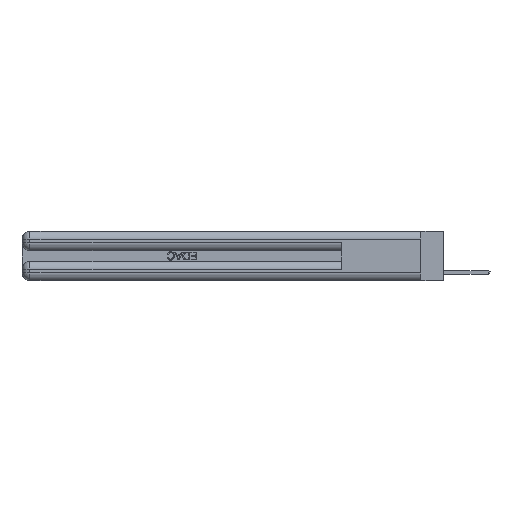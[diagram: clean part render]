
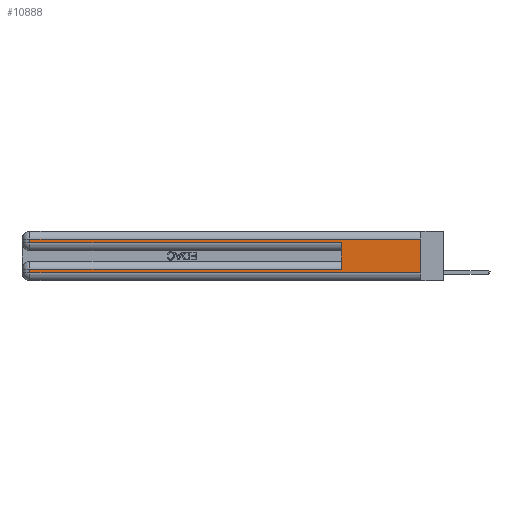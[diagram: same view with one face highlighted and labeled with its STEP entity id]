
A CAD part, left-side view. The second image highlights one B-rep face of the part: STEP entity #10888.
In plain terms, the highlighted planar face has unit normal (-1, 0, 0).
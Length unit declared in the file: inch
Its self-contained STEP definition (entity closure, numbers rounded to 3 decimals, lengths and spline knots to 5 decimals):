
#2613 = ORIENTED_EDGE ( 'NONE', *, *, #18025, .T. ) ;
#2852 = CARTESIAN_POINT ( 'NONE',  ( 0., 0., 0.31 ) ) ;
#3670 = VERTEX_POINT ( 'NONE', #18301 ) ;
#3896 = CARTESIAN_POINT ( 'NONE',  ( 0., 0., 0.31 ) ) ;
#4513 = VECTOR ( 'NONE', #7351, 39.37008 ) ;
#4706 = FACE_OUTER_BOUND ( 'NONE', #17770, .T. ) ;
#5060 = CARTESIAN_POINT ( 'NONE',  ( 0., 0., 0.06 ) ) ;
#5392 = VERTEX_POINT ( 'NONE', #24431 ) ;
#6036 = VERTEX_POINT ( 'NONE', #26670 ) ;
#6411 = VERTEX_POINT ( 'NONE', #17900 ) ;
#6585 = CARTESIAN_POINT ( 'NONE',  ( 0., 0.6, 0.145 ) ) ;
#7351 = DIRECTION ( 'NONE',  ( 0., 0., -1. ) ) ;
#8459 = ORIENTED_EDGE ( 'NONE', *, *, #19089, .F. ) ;
#9196 = CARTESIAN_POINT ( 'NONE',  ( 0., 2.94, 0.085 ) ) ;
#10409 = DIRECTION ( 'NONE',  ( 0., 0., -1. ) ) ;
#10888 = ADVANCED_FACE ( 'NONE', ( #4706 ), #28936, .F. ) ;
#11468 = LINE ( 'NONE', #24346, #15076 ) ;
#11641 = DIRECTION ( 'NONE',  ( 0., -1., 0. ) ) ;
#11664 = EDGE_CURVE ( 'NONE', #6036, #26321, #22781, .T. ) ;
#12719 = VECTOR ( 'NONE', #18412, 39.37008 ) ;
#12930 = AXIS2_PLACEMENT_3D ( 'NONE', #17238, #15119, #26695 ) ;
#13207 = ORIENTED_EDGE ( 'NONE', *, *, #11664, .T. ) ;
#13581 = LINE ( 'NONE', #27508, #18640 ) ;
#13871 = VECTOR ( 'NONE', #19213, 39.37008 ) ;
#14738 = CARTESIAN_POINT ( 'NONE',  ( 0., 2.94, 0.37 ) ) ;
#15076 = VECTOR ( 'NONE', #10409, 39.37008 ) ;
#15119 = DIRECTION ( 'NONE',  ( 1., 0., 0. ) ) ;
#16071 = ORIENTED_EDGE ( 'NONE', *, *, #19664, .T. ) ;
#16158 = EDGE_CURVE ( 'NONE', #26321, #28651, #26924, .T. ) ;
#16283 = VERTEX_POINT ( 'NONE', #20315 ) ;
#16354 = ORIENTED_EDGE ( 'NONE', *, *, #24091, .T. ) ;
#16375 = ORIENTED_EDGE ( 'NONE', *, *, #16158, .T. ) ;
#17210 = DIRECTION ( 'NONE',  ( 0., 1., 0. ) ) ;
#17238 = CARTESIAN_POINT ( 'NONE',  ( 0., 0., 0.37 ) ) ;
#17770 = EDGE_LOOP ( 'NONE', ( #19878, #16071, #16354, #28757, #8459, #13207, #16375, #2613 ) ) ;
#17900 = CARTESIAN_POINT ( 'NONE',  ( 0., 2.94, 0.285 ) ) ;
#18025 = EDGE_CURVE ( 'NONE', #28651, #16283, #19269, .T. ) ;
#18301 = CARTESIAN_POINT ( 'NONE',  ( 0., 0.6, 0.285 ) ) ;
#18412 = DIRECTION ( 'NONE',  ( 0., 0., 1. ) ) ;
#18640 = VECTOR ( 'NONE', #23364, 39.37008 ) ;
#19089 = EDGE_CURVE ( 'NONE', #6036, #3670, #21743, .T. ) ;
#19213 = DIRECTION ( 'NONE',  ( 0., 1., 0. ) ) ;
#19269 = LINE ( 'NONE', #5060, #20688 ) ;
#19350 = DIRECTION ( 'NONE',  ( 0., -1., 0. ) ) ;
#19601 = VECTOR ( 'NONE', #11641, 39.37008 ) ;
#19664 = EDGE_CURVE ( 'NONE', #20798, #5392, #20693, .T. ) ;
#19878 = ORIENTED_EDGE ( 'NONE', *, *, #28445, .F. ) ;
#20315 = CARTESIAN_POINT ( 'NONE',  ( 0., 0., 0.06 ) ) ;
#20688 = VECTOR ( 'NONE', #19350, 39.37008 ) ;
#20693 = LINE ( 'NONE', #2852, #13871 ) ;
#20798 = VERTEX_POINT ( 'NONE', #3896 ) ;
#21138 = EDGE_CURVE ( 'NONE', #6411, #3670, #25729, .T. ) ;
#21698 = VECTOR ( 'NONE', #17210, 39.37008 ) ;
#21743 = LINE ( 'NONE', #6585, #12719 ) ;
#22781 = LINE ( 'NONE', #28808, #21698 ) ;
#23146 = CARTESIAN_POINT ( 'NONE',  ( 0., 0., 0.285 ) ) ;
#23364 = DIRECTION ( 'NONE',  ( 0., 0., -1. ) ) ;
#24091 = EDGE_CURVE ( 'NONE', #5392, #6411, #11468, .T. ) ;
#24346 = CARTESIAN_POINT ( 'NONE',  ( 0., 2.94, 0.37 ) ) ;
#24431 = CARTESIAN_POINT ( 'NONE',  ( 0., 2.94, 0.31 ) ) ;
#25729 = LINE ( 'NONE', #23146, #19601 ) ;
#26321 = VERTEX_POINT ( 'NONE', #9196 ) ;
#26670 = CARTESIAN_POINT ( 'NONE',  ( 0., 0.6, 0.085 ) ) ;
#26695 = DIRECTION ( 'NONE',  ( 0., 0., -1. ) ) ;
#26924 = LINE ( 'NONE', #14738, #4513 ) ;
#27508 = CARTESIAN_POINT ( 'NONE',  ( 0., 0., 0.37 ) ) ;
#28445 = EDGE_CURVE ( 'NONE', #20798, #16283, #13581, .T. ) ;
#28524 = CARTESIAN_POINT ( 'NONE',  ( 0., 2.94, 0.06 ) ) ;
#28651 = VERTEX_POINT ( 'NONE', #28524 ) ;
#28757 = ORIENTED_EDGE ( 'NONE', *, *, #21138, .T. ) ;
#28808 = CARTESIAN_POINT ( 'NONE',  ( 0., 0., 0.085 ) ) ;
#28936 = PLANE ( 'NONE',  #12930 ) ;
